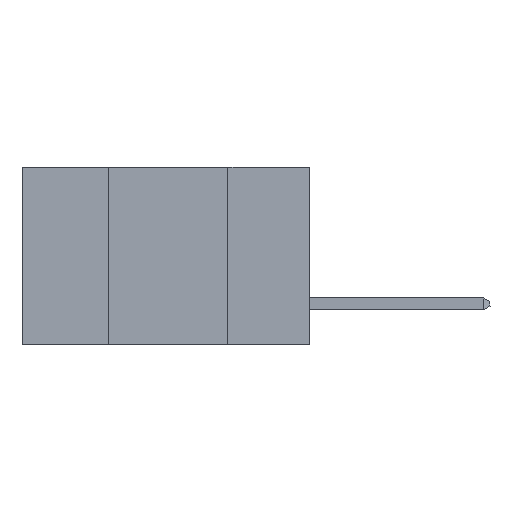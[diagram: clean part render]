
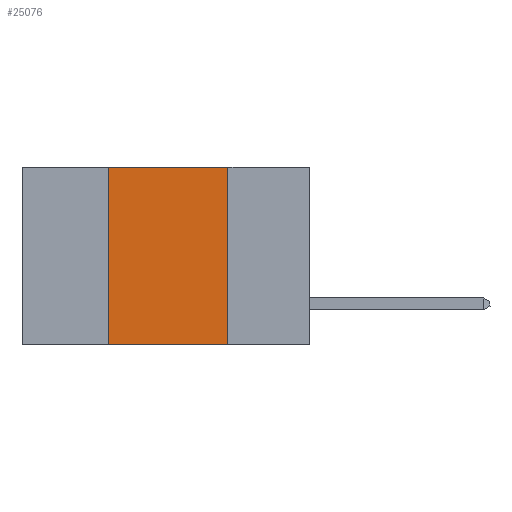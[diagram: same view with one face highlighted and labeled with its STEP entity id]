
A CAD part, left-side view. The second image highlights one B-rep face of the part: STEP entity #25076.
In plain terms, the highlighted planar face has unit normal (-1, 0, 0).
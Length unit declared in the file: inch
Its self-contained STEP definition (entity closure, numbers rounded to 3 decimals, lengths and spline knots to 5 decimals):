
#167 = VECTOR ( 'NONE', #21773, 39.37008 ) ;
#617 = VECTOR ( 'NONE', #629, 39.37008 ) ;
#629 = DIRECTION ( 'NONE',  ( 0., 0., -1. ) ) ;
#686 = CARTESIAN_POINT ( 'NONE',  ( 0., 0.17, -0.37 ) ) ;
#787 = CARTESIAN_POINT ( 'NONE',  ( 0., 0.6, 0. ) ) ;
#2189 = FACE_OUTER_BOUND ( 'NONE', #15409, .T. ) ;
#2239 = ORIENTED_EDGE ( 'NONE', *, *, #22270, .F. ) ;
#2613 = EDGE_CURVE ( 'NONE', #16626, #3325, #14107, .T. ) ;
#2684 = LINE ( 'NONE', #23782, #7582 ) ;
#2919 = ORIENTED_EDGE ( 'NONE', *, *, #25135, .T. ) ;
#3325 = VERTEX_POINT ( 'NONE', #15516 ) ;
#4467 = ORIENTED_EDGE ( 'NONE', *, *, #22751, .F. ) ;
#4804 = CARTESIAN_POINT ( 'NONE',  ( 0., 0.17, 0. ) ) ;
#5133 = DIRECTION ( 'NONE',  ( 0., 0., -1. ) ) ;
#5930 = VERTEX_POINT ( 'NONE', #686 ) ;
#6258 = LINE ( 'NONE', #4804, #617 ) ;
#6458 = LINE ( 'NONE', #21865, #167 ) ;
#7582 = VECTOR ( 'NONE', #15685, 39.37008 ) ;
#10756 = VERTEX_POINT ( 'NONE', #21018 ) ;
#11577 = CARTESIAN_POINT ( 'NONE',  ( 0., 0.42, 0. ) ) ;
#11662 = DIRECTION ( 'NONE',  ( 0., 0., 1. ) ) ;
#13345 = ORIENTED_EDGE ( 'NONE', *, *, #2613, .F. ) ;
#14107 = LINE ( 'NONE', #11577, #19600 ) ;
#15409 = EDGE_LOOP ( 'NONE', ( #4467, #2239, #13345, #2919 ) ) ;
#15516 = CARTESIAN_POINT ( 'NONE',  ( 0., 0.42, 0. ) ) ;
#15527 = PLANE ( 'NONE',  #17198 ) ;
#15685 = DIRECTION ( 'NONE',  ( 0., -1., 0. ) ) ;
#16626 = VERTEX_POINT ( 'NONE', #20317 ) ;
#17198 = AXIS2_PLACEMENT_3D ( 'NONE', #787, #17580, #5133 ) ;
#17580 = DIRECTION ( 'NONE',  ( 1., 0., 0. ) ) ;
#19600 = VECTOR ( 'NONE', #11662, 39.37008 ) ;
#20317 = CARTESIAN_POINT ( 'NONE',  ( 0., 0.42, -0.37 ) ) ;
#21018 = CARTESIAN_POINT ( 'NONE',  ( 0., 0.17, 0. ) ) ;
#21773 = DIRECTION ( 'NONE',  ( 0., -1., 0. ) ) ;
#21865 = CARTESIAN_POINT ( 'NONE',  ( 0., 0.6, -0.37 ) ) ;
#22270 = EDGE_CURVE ( 'NONE', #3325, #10756, #2684, .T. ) ;
#22751 = EDGE_CURVE ( 'NONE', #10756, #5930, #6258, .T. ) ;
#23782 = CARTESIAN_POINT ( 'NONE',  ( 0., 0.6, 0. ) ) ;
#25076 = ADVANCED_FACE ( 'NONE', ( #2189 ), #15527, .F. ) ;
#25135 = EDGE_CURVE ( 'NONE', #16626, #5930, #6458, .T. ) ;
